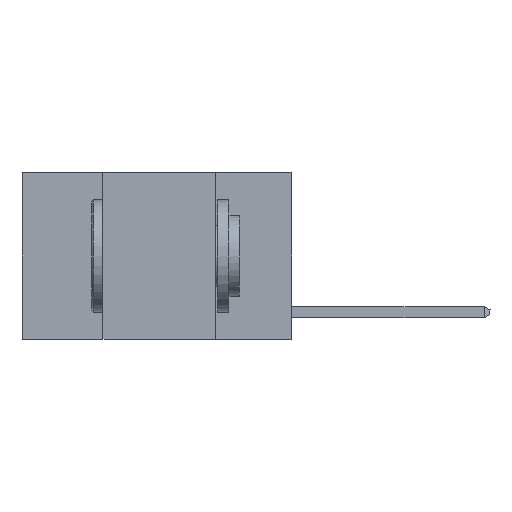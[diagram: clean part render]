
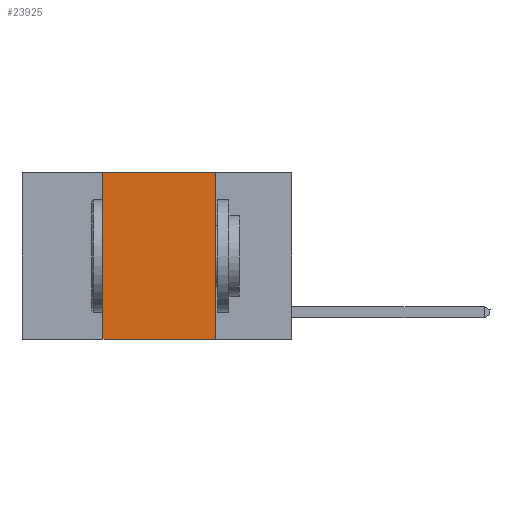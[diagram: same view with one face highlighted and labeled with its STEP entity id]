
A CAD part, left-side view. The second image highlights one B-rep face of the part: STEP entity #23925.
In plain terms, the highlighted planar face has unit normal (-1, 0, 0).
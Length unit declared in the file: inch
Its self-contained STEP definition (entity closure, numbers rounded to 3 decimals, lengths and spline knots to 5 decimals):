
#466 = EDGE_CURVE ( 'NONE', #17152, #22603, #8209, .T. ) ;
#764 = CARTESIAN_POINT ( 'NONE',  ( 0., 0.17, 0. ) ) ;
#1123 = CARTESIAN_POINT ( 'NONE',  ( 0., 0.42, 0. ) ) ;
#1721 = DIRECTION ( 'NONE',  ( 0., -1., 0. ) ) ;
#1879 = DIRECTION ( 'NONE',  ( 0., 0., -1. ) ) ;
#3936 = CARTESIAN_POINT ( 'NONE',  ( 0., 0.17, 0. ) ) ;
#5596 = EDGE_CURVE ( 'NONE', #22603, #20971, #19576, .T. ) ;
#5934 = ORIENTED_EDGE ( 'NONE', *, *, #466, .F. ) ;
#6303 = PLANE ( 'NONE',  #17760 ) ;
#7762 = VECTOR ( 'NONE', #1721, 39.37008 ) ;
#7845 = CARTESIAN_POINT ( 'NONE',  ( 0., 0.42, -0.37 ) ) ;
#8209 = LINE ( 'NONE', #15415, #25212 ) ;
#8393 = CARTESIAN_POINT ( 'NONE',  ( 0., 0.6, -0.37 ) ) ;
#8469 = VECTOR ( 'NONE', #9650, 39.37008 ) ;
#9650 = DIRECTION ( 'NONE',  ( 0., 0., -1. ) ) ;
#11903 = VERTEX_POINT ( 'NONE', #7845 ) ;
#12161 = DIRECTION ( 'NONE',  ( 0., 0., 1. ) ) ;
#12924 = ORIENTED_EDGE ( 'NONE', *, *, #5596, .F. ) ;
#13545 = FACE_OUTER_BOUND ( 'NONE', #28600, .T. ) ;
#13688 = LINE ( 'NONE', #8393, #7762 ) ;
#15235 = DIRECTION ( 'NONE',  ( 1., 0., 0. ) ) ;
#15314 = DIRECTION ( 'NONE',  ( 0., -1., 0. ) ) ;
#15415 = CARTESIAN_POINT ( 'NONE',  ( 0., 0.6, 0. ) ) ;
#16239 = VECTOR ( 'NONE', #12161, 39.37008 ) ;
#17152 = VERTEX_POINT ( 'NONE', #26715 ) ;
#17475 = EDGE_CURVE ( 'NONE', #11903, #17152, #28023, .T. ) ;
#17760 = AXIS2_PLACEMENT_3D ( 'NONE', #28516, #15235, #1879 ) ;
#19576 = LINE ( 'NONE', #764, #8469 ) ;
#20971 = VERTEX_POINT ( 'NONE', #28231 ) ;
#21669 = ORIENTED_EDGE ( 'NONE', *, *, #17475, .F. ) ;
#22603 = VERTEX_POINT ( 'NONE', #3936 ) ;
#23010 = ORIENTED_EDGE ( 'NONE', *, *, #23254, .T. ) ;
#23254 = EDGE_CURVE ( 'NONE', #11903, #20971, #13688, .T. ) ;
#23925 = ADVANCED_FACE ( 'NONE', ( #13545 ), #6303, .F. ) ;
#25212 = VECTOR ( 'NONE', #15314, 39.37008 ) ;
#26715 = CARTESIAN_POINT ( 'NONE',  ( 0., 0.42, 0. ) ) ;
#28023 = LINE ( 'NONE', #1123, #16239 ) ;
#28231 = CARTESIAN_POINT ( 'NONE',  ( 0., 0.17, -0.37 ) ) ;
#28516 = CARTESIAN_POINT ( 'NONE',  ( 0., 0.6, 0. ) ) ;
#28600 = EDGE_LOOP ( 'NONE', ( #12924, #5934, #21669, #23010 ) ) ;
